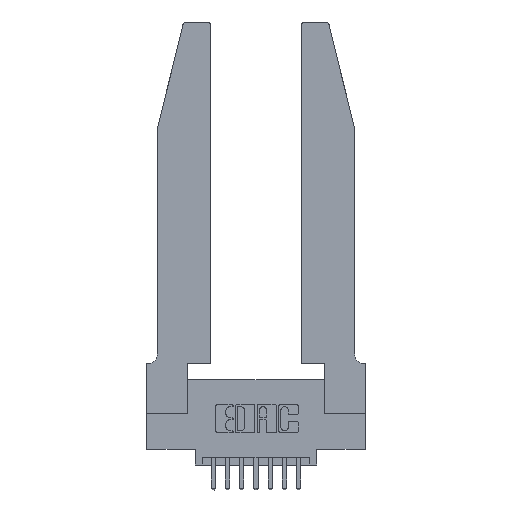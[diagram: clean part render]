
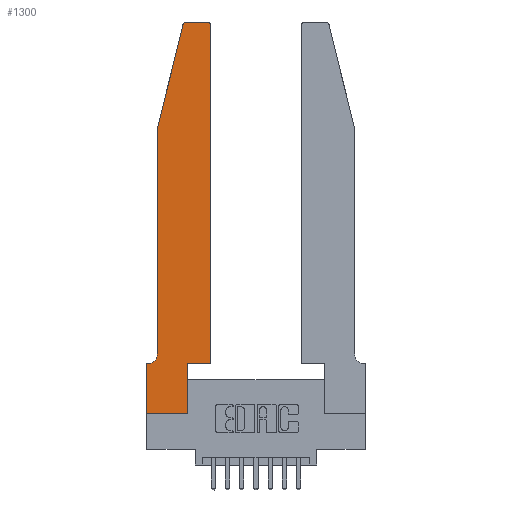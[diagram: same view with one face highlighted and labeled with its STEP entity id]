
A CAD part, top view. The second image highlights one B-rep face of the part: STEP entity #1300.
In plain terms, the highlighted planar face has unit normal (0, 0, 1).
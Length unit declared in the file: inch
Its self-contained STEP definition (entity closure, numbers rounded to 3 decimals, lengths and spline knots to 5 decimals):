
#80 = DIRECTION ( 'NONE',  ( -0.239, -0.971, 0. ) ) ;
#100 = DIRECTION ( 'NONE',  ( 1., 0., 0. ) ) ;
#407 = CARTESIAN_POINT ( 'NONE',  ( 0.4505, 0.35, 0.37 ) ) ;
#434 = DIRECTION ( 'NONE',  ( 0., -1., 0. ) ) ;
#1006 = VERTEX_POINT ( 'NONE', #4512 ) ;
#1109 = ORIENTED_EDGE ( 'NONE', *, *, #7837, .T. ) ;
#1195 = DIRECTION ( 'NONE',  ( 0., -1., 0. ) ) ;
#1232 = LINE ( 'NONE', #12920, #14628 ) ;
#1300 = ADVANCED_FACE ( 'NONE', ( #11590 ), #5398, .T. ) ;
#1362 = EDGE_CURVE ( 'NONE', #12231, #6291, #7165, .T. ) ;
#1387 = EDGE_CURVE ( 'NONE', #3231, #4661, #11766, .T. ) ;
#1609 = DIRECTION ( 'NONE',  ( -1., 0., 0. ) ) ;
#1767 = EDGE_CURVE ( 'NONE', #13897, #1006, #4772, .T. ) ;
#1927 = DIRECTION ( 'NONE',  ( 0., 0., 1. ) ) ;
#1958 = CARTESIAN_POINT ( 'NONE',  ( 0.0755, 0.42, 0.37 ) ) ;
#1960 = ORIENTED_EDGE ( 'NONE', *, *, #1362, .T. ) ;
#2069 = CARTESIAN_POINT ( 'NONE',  ( 0.25487, 2.72718, 0.37 ) ) ;
#2120 = CARTESIAN_POINT ( 'NONE',  ( 0., 0.35, 0.37 ) ) ;
#2192 = CARTESIAN_POINT ( 'NONE',  ( 0.4505, 0.35, 0.37 ) ) ;
#2201 = DIRECTION ( 'NONE',  ( 1., 0., 0. ) ) ;
#2879 = DIRECTION ( 'NONE',  ( 1., 0., 0. ) ) ;
#2907 = EDGE_CURVE ( 'NONE', #4661, #4211, #2909, .T. ) ;
#2909 = LINE ( 'NONE', #3684, #13006 ) ;
#2916 = EDGE_CURVE ( 'NONE', #9438, #3231, #5656, .T. ) ;
#2993 = VERTEX_POINT ( 'NONE', #4884 ) ;
#3231 = VERTEX_POINT ( 'NONE', #1958 ) ;
#3451 = ORIENTED_EDGE ( 'NONE', *, *, #5865, .T. ) ;
#3558 = EDGE_CURVE ( 'NONE', #2993, #12231, #8557, .T. ) ;
#3584 = LINE ( 'NONE', #13837, #10363 ) ;
#3607 = DIRECTION ( 'NONE',  ( 0., 1., 0. ) ) ;
#3620 = LINE ( 'NONE', #12962, #13331 ) ;
#3640 = ORIENTED_EDGE ( 'NONE', *, *, #5384, .T. ) ;
#3650 = LINE ( 'NONE', #13717, #14882 ) ;
#3684 = CARTESIAN_POINT ( 'NONE',  ( 0.0755, 0.35, 0.37 ) ) ;
#3962 = DIRECTION ( 'NONE',  ( 0., 0., -1. ) ) ;
#4211 = VERTEX_POINT ( 'NONE', #2120 ) ;
#4277 = DIRECTION ( 'NONE',  ( 1., 0., 0. ) ) ;
#4297 = CARTESIAN_POINT ( 'NONE',  ( 0.4505, 0.35, 0.37 ) ) ;
#4403 = DIRECTION ( 'NONE',  ( 0., 1., 0. ) ) ;
#4512 = CARTESIAN_POINT ( 'NONE',  ( 0.284, 2.75, 0.37 ) ) ;
#4661 = VERTEX_POINT ( 'NONE', #10503 ) ;
#4726 = ORIENTED_EDGE ( 'NONE', *, *, #2916, .T. ) ;
#4744 = VECTOR ( 'NONE', #1195, 39.37008 ) ;
#4772 = LINE ( 'NONE', #8713, #10084 ) ;
#4884 = CARTESIAN_POINT ( 'NONE',  ( 0.2865, 0.35, 0.37 ) ) ;
#5156 = CARTESIAN_POINT ( 'NONE',  ( 0.4205, 2.72, 0.37 ) ) ;
#5170 = CARTESIAN_POINT ( 'NONE',  ( 0.2865, 0., 0.37 ) ) ;
#5366 = CIRCLE ( 'NONE', #9392, 0.03 ) ;
#5383 = ORIENTED_EDGE ( 'NONE', *, *, #2907, .T. ) ;
#5384 = EDGE_CURVE ( 'NONE', #4211, #7754, #3620, .T. ) ;
#5398 = PLANE ( 'NONE',  #8378 ) ;
#5656 = LINE ( 'NONE', #6052, #4744 ) ;
#5865 = EDGE_CURVE ( 'NONE', #7414, #9438, #1232, .T. ) ;
#5938 = ORIENTED_EDGE ( 'NONE', *, *, #6886, .T. ) ;
#6052 = CARTESIAN_POINT ( 'NONE',  ( 0.0755, 2., 0.37 ) ) ;
#6176 = ORIENTED_EDGE ( 'NONE', *, *, #3558, .T. ) ;
#6291 = VERTEX_POINT ( 'NONE', #9534 ) ;
#6497 = AXIS2_PLACEMENT_3D ( 'NONE', #10473, #9401, #100 ) ;
#6541 = AXIS2_PLACEMENT_3D ( 'NONE', #10583, #3962, #1609 ) ;
#6643 = CARTESIAN_POINT ( 'NONE',  ( 0., 0.35, 0.37 ) ) ;
#6877 = CARTESIAN_POINT ( 'NONE',  ( 0.4205, 2.75, 0.37 ) ) ;
#6886 = EDGE_CURVE ( 'NONE', #7754, #7021, #3584, .T. ) ;
#7021 = VERTEX_POINT ( 'NONE', #5170 ) ;
#7165 = LINE ( 'NONE', #4297, #8088 ) ;
#7397 = DIRECTION ( 'NONE',  ( 0., 0., 1. ) ) ;
#7414 = VERTEX_POINT ( 'NONE', #2069 ) ;
#7754 = VERTEX_POINT ( 'NONE', #13858 ) ;
#7837 = EDGE_CURVE ( 'NONE', #6291, #13897, #5366, .T. ) ;
#7862 = ORIENTED_EDGE ( 'NONE', *, *, #12438, .T. ) ;
#8088 = VECTOR ( 'NONE', #4403, 39.37008 ) ;
#8107 = CIRCLE ( 'NONE', #6497, 0.03 ) ;
#8378 = AXIS2_PLACEMENT_3D ( 'NONE', #6643, #1927, #4277 ) ;
#8557 = LINE ( 'NONE', #407, #13527 ) ;
#8713 = CARTESIAN_POINT ( 'NONE',  ( 0.2605, 2.75, 0.37 ) ) ;
#8768 = DIRECTION ( 'NONE',  ( -1., 0., 0. ) ) ;
#9047 = EDGE_LOOP ( 'NONE', ( #9849, #7862, #3451, #4726, #9910, #5383, #3640, #5938, #13654, #6176, #1960, #1109 ) ) ;
#9392 = AXIS2_PLACEMENT_3D ( 'NONE', #5156, #7397, #13349 ) ;
#9401 = DIRECTION ( 'NONE',  ( 0., 0., 1. ) ) ;
#9438 = VERTEX_POINT ( 'NONE', #11151 ) ;
#9534 = CARTESIAN_POINT ( 'NONE',  ( 0.4505, 2.72, 0.37 ) ) ;
#9849 = ORIENTED_EDGE ( 'NONE', *, *, #1767, .T. ) ;
#9910 = ORIENTED_EDGE ( 'NONE', *, *, #1387, .T. ) ;
#10084 = VECTOR ( 'NONE', #8768, 39.37008 ) ;
#10363 = VECTOR ( 'NONE', #2201, 39.37008 ) ;
#10473 = CARTESIAN_POINT ( 'NONE',  ( 0.284, 2.72, 0.37 ) ) ;
#10503 = CARTESIAN_POINT ( 'NONE',  ( 0.0055, 0.35, 0.37 ) ) ;
#10583 = CARTESIAN_POINT ( 'NONE',  ( 0.0055, 0.42, 0.37 ) ) ;
#11151 = CARTESIAN_POINT ( 'NONE',  ( 0.0755, 2., 0.37 ) ) ;
#11590 = FACE_OUTER_BOUND ( 'NONE', #9047, .T. ) ;
#11766 = CIRCLE ( 'NONE', #6541, 0.07 ) ;
#12231 = VERTEX_POINT ( 'NONE', #2192 ) ;
#12438 = EDGE_CURVE ( 'NONE', #1006, #7414, #8107, .T. ) ;
#12920 = CARTESIAN_POINT ( 'NONE',  ( 0.0755, 2., 0.37 ) ) ;
#12962 = CARTESIAN_POINT ( 'NONE',  ( 0., 0., 0.37 ) ) ;
#13006 = VECTOR ( 'NONE', #13024, 39.37008 ) ;
#13024 = DIRECTION ( 'NONE',  ( -1., 0., 0. ) ) ;
#13331 = VECTOR ( 'NONE', #434, 39.37008 ) ;
#13349 = DIRECTION ( 'NONE',  ( 1., 0., 0. ) ) ;
#13527 = VECTOR ( 'NONE', #2879, 39.37008 ) ;
#13654 = ORIENTED_EDGE ( 'NONE', *, *, #14131, .T. ) ;
#13717 = CARTESIAN_POINT ( 'NONE',  ( 0.2865, 0.35, 0.37 ) ) ;
#13837 = CARTESIAN_POINT ( 'NONE',  ( 0., 0., 0.37 ) ) ;
#13858 = CARTESIAN_POINT ( 'NONE',  ( 0., 0., 0.37 ) ) ;
#13897 = VERTEX_POINT ( 'NONE', #6877 ) ;
#14131 = EDGE_CURVE ( 'NONE', #7021, #2993, #3650, .T. ) ;
#14628 = VECTOR ( 'NONE', #80, 39.37008 ) ;
#14882 = VECTOR ( 'NONE', #3607, 39.37008 ) ;
